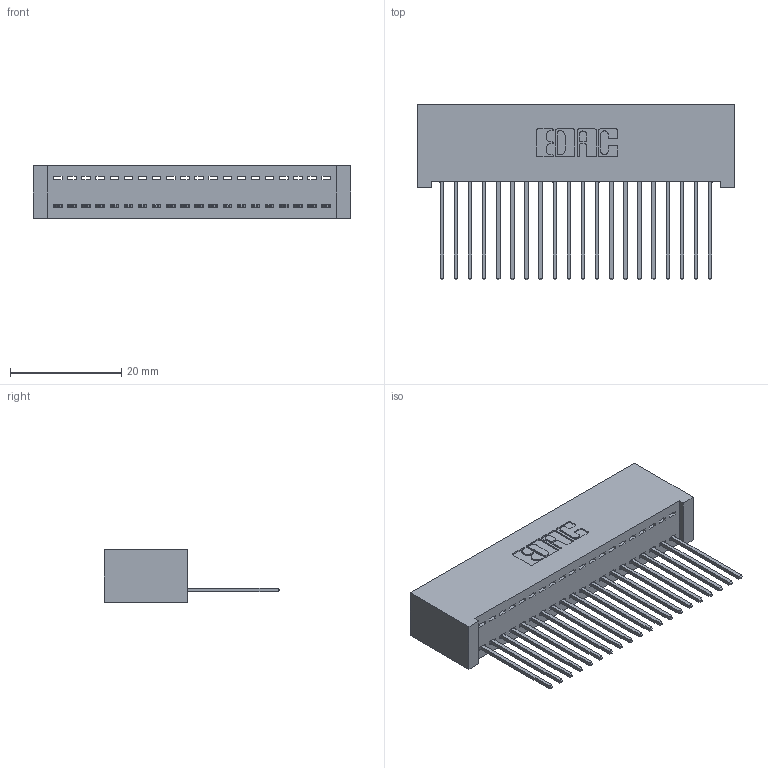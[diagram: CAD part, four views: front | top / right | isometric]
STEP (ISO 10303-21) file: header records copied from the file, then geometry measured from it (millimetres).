
FILE_DESCRIPTION (( 'STEP AP203' ), '1' );
FILE_NAME ('342-020-542-101.STEP', '2019-10-01T21:14:51', ( '' ), ( '' ), 'SwSTEP 2.0', 'SolidWorks 2016', '' );
FILE_SCHEMA (( 'CONFIG_CONTROL_DESIGN' ));
Length unit declared in the file: inch
Products named in the file (3): 342 Part_Lugless; 345-292-001_345-293-142; 342-020-542-101
Assembly tree (21 placements, depth 2):
  342-020-542-101
    342 Part_Lugless
    345-292-001_345-293-142  x20
Bounding box: 57.05 x 31.63 x 9.4 mm (x, y, z)
Volume: 5374.4 mm3; surface area: 8076 mm2
Topology: 21 solids, 21 shells, 1262 faces, 3795 edges, 2502 vertices
Faces by surface type: plane 902, cylinder 360
Entity records: 14681 total; most frequent: CARTESIAN_POINT 2542, ORIENTED_EDGE 2498, DIRECTION 2181, EDGE_CURVE 1249, LINE 1129, VECTOR 1129, VERTEX_POINT 830, AXIS2_PLACEMENT_3D 526
